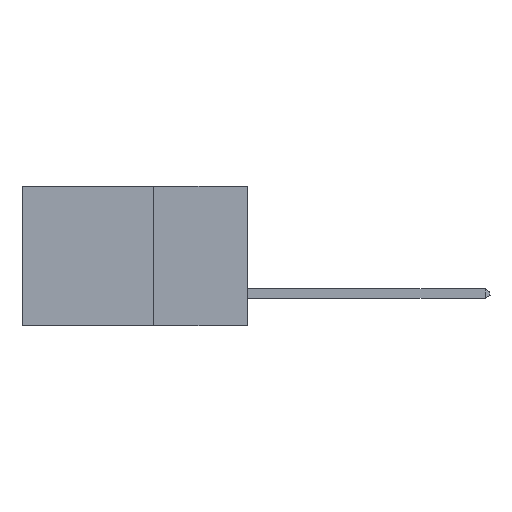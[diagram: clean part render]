
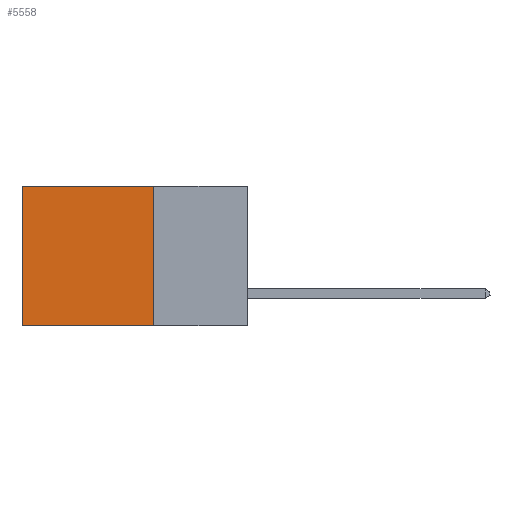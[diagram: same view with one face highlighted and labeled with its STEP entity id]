
A CAD part, left-side view. The second image highlights one B-rep face of the part: STEP entity #5558.
In plain terms, the highlighted planar face has unit normal (-1, 0, 0).
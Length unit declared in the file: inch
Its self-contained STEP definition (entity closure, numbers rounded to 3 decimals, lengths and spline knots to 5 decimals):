
#1371 = LINE ( 'NONE', #12059, #13670 ) ;
#1588 = DIRECTION ( 'NONE',  ( 0., 0., -1. ) ) ;
#1879 = CARTESIAN_POINT ( 'NONE',  ( 0.298, 0.25, 0. ) ) ;
#2002 = VECTOR ( 'NONE', #1588, 39.37008 ) ;
#2393 = LINE ( 'NONE', #8934, #2002 ) ;
#2497 = CARTESIAN_POINT ( 'NONE',  ( 0.298, 0.25, -0.37 ) ) ;
#3228 = DIRECTION ( 'NONE',  ( 1., 0., 0. ) ) ;
#3415 = LINE ( 'NONE', #10337, #13595 ) ;
#4329 = CARTESIAN_POINT ( 'NONE',  ( 0.298, 0.6, -0.37 ) ) ;
#5060 = ORIENTED_EDGE ( 'NONE', *, *, #7021, .T. ) ;
#5098 = ORIENTED_EDGE ( 'NONE', *, *, #12548, .T. ) ;
#5155 = EDGE_LOOP ( 'NONE', ( #5060, #15406, #15570, #5098 ) ) ;
#5242 = CARTESIAN_POINT ( 'NONE',  ( 0.298, 0.6, 0. ) ) ;
#5467 = EDGE_CURVE ( 'NONE', #8580, #10120, #3415, .T. ) ;
#5558 = ADVANCED_FACE ( 'NONE', ( #7622 ), #9180, .F. ) ;
#6951 = VERTEX_POINT ( 'NONE', #5242 ) ;
#7021 = EDGE_CURVE ( 'NONE', #6951, #10120, #2393, .T. ) ;
#7622 = FACE_OUTER_BOUND ( 'NONE', #5155, .T. ) ;
#8580 = VERTEX_POINT ( 'NONE', #2497 ) ;
#8934 = CARTESIAN_POINT ( 'NONE',  ( 0.298, 0.6, 0. ) ) ;
#9013 = VECTOR ( 'NONE', #11940, 39.37008 ) ;
#9180 = PLANE ( 'NONE',  #14030 ) ;
#9266 = EDGE_CURVE ( 'NONE', #14043, #8580, #1371, .T. ) ;
#10120 = VERTEX_POINT ( 'NONE', #4329 ) ;
#10337 = CARTESIAN_POINT ( 'NONE',  ( 0.298, 0.25, -0.37 ) ) ;
#11610 = DIRECTION ( 'NONE',  ( 0., 0., -1. ) ) ;
#11801 = CARTESIAN_POINT ( 'NONE',  ( 0.298, 0.25, 0. ) ) ;
#11940 = DIRECTION ( 'NONE',  ( 0., 1., 0. ) ) ;
#12006 = DIRECTION ( 'NONE',  ( 0., 0., -1. ) ) ;
#12059 = CARTESIAN_POINT ( 'NONE',  ( 0.298, 0.25, 0. ) ) ;
#12548 = EDGE_CURVE ( 'NONE', #14043, #6951, #15175, .T. ) ;
#13595 = VECTOR ( 'NONE', #14047, 39.37008 ) ;
#13670 = VECTOR ( 'NONE', #12006, 39.37008 ) ;
#14030 = AXIS2_PLACEMENT_3D ( 'NONE', #1879, #3228, #11610 ) ;
#14043 = VERTEX_POINT ( 'NONE', #11801 ) ;
#14047 = DIRECTION ( 'NONE',  ( 0., 1., 0. ) ) ;
#14461 = CARTESIAN_POINT ( 'NONE',  ( 0.298, 0.25, 0. ) ) ;
#15175 = LINE ( 'NONE', #14461, #9013 ) ;
#15406 = ORIENTED_EDGE ( 'NONE', *, *, #5467, .F. ) ;
#15570 = ORIENTED_EDGE ( 'NONE', *, *, #9266, .F. ) ;
